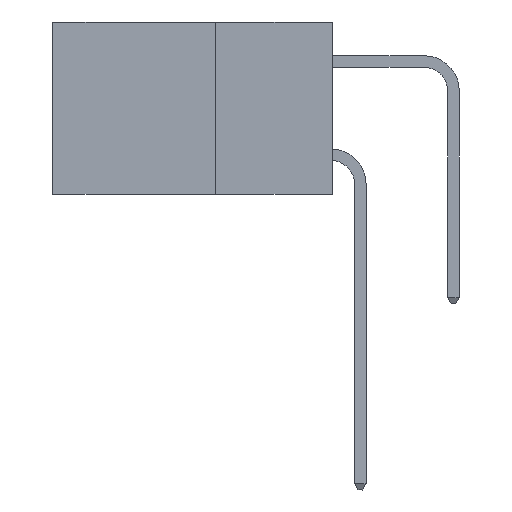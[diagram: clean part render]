
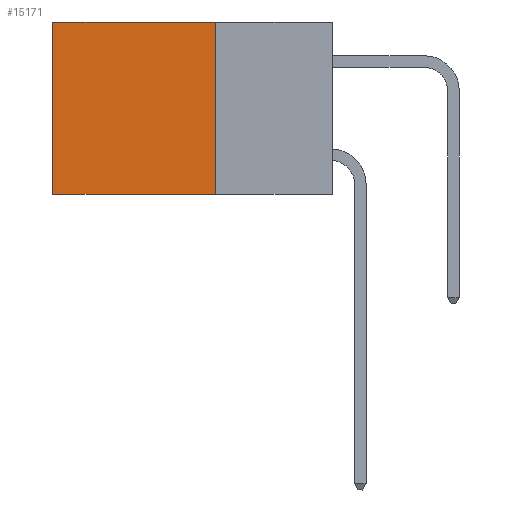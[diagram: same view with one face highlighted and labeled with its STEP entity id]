
A CAD part, left-side view. The second image highlights one B-rep face of the part: STEP entity #15171.
In plain terms, the highlighted planar face has unit normal (-1, 0, 0).
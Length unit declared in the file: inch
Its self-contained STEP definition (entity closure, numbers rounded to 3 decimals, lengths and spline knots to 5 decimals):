
#57 = DIRECTION ( 'NONE',  ( 0., 1., 0. ) ) ;
#191 = CARTESIAN_POINT ( 'NONE',  ( 0.298, 0.25, 0. ) ) ;
#913 = EDGE_CURVE ( 'NONE', #8604, #12734, #20080, .T. ) ;
#1960 = DIRECTION ( 'NONE',  ( 0., 1., 0. ) ) ;
#3022 = ORIENTED_EDGE ( 'NONE', *, *, #7947, .T. ) ;
#3109 = CARTESIAN_POINT ( 'NONE',  ( 0.298, 0.25, 0. ) ) ;
#3699 = VERTEX_POINT ( 'NONE', #13291 ) ;
#3795 = ORIENTED_EDGE ( 'NONE', *, *, #8197, .F. ) ;
#5939 = VERTEX_POINT ( 'NONE', #18798 ) ;
#6107 = LINE ( 'NONE', #9723, #14970 ) ;
#6274 = DIRECTION ( 'NONE',  ( 1., 0., 0. ) ) ;
#7087 = VECTOR ( 'NONE', #57, 39.37008 ) ;
#7766 = PLANE ( 'NONE',  #12631 ) ;
#7947 = EDGE_CURVE ( 'NONE', #5939, #8604, #10801, .T. ) ;
#8197 = EDGE_CURVE ( 'NONE', #5939, #3699, #9546, .T. ) ;
#8595 = EDGE_LOOP ( 'NONE', ( #16766, #17798, #3795, #3022 ) ) ;
#8604 = VERTEX_POINT ( 'NONE', #13914 ) ;
#8838 = EDGE_CURVE ( 'NONE', #3699, #12734, #6107, .T. ) ;
#9516 = CARTESIAN_POINT ( 'NONE',  ( 0.298, 0.6, 0. ) ) ;
#9546 = LINE ( 'NONE', #191, #17985 ) ;
#9723 = CARTESIAN_POINT ( 'NONE',  ( 0.298, 0.25, -0.37 ) ) ;
#9848 = CARTESIAN_POINT ( 'NONE',  ( 0.298, 0.25, 0. ) ) ;
#10801 = LINE ( 'NONE', #9848, #7087 ) ;
#11315 = VECTOR ( 'NONE', #18685, 39.37008 ) ;
#11689 = FACE_OUTER_BOUND ( 'NONE', #8595, .T. ) ;
#12631 = AXIS2_PLACEMENT_3D ( 'NONE', #3109, #6274, #17336 ) ;
#12734 = VERTEX_POINT ( 'NONE', #17383 ) ;
#13291 = CARTESIAN_POINT ( 'NONE',  ( 0.298, 0.25, -0.37 ) ) ;
#13914 = CARTESIAN_POINT ( 'NONE',  ( 0.298, 0.6, 0. ) ) ;
#14970 = VECTOR ( 'NONE', #1960, 39.37008 ) ;
#15171 = ADVANCED_FACE ( 'NONE', ( #11689 ), #7766, .F. ) ;
#15884 = DIRECTION ( 'NONE',  ( 0., 0., -1. ) ) ;
#16766 = ORIENTED_EDGE ( 'NONE', *, *, #913, .T. ) ;
#17336 = DIRECTION ( 'NONE',  ( 0., 0., -1. ) ) ;
#17383 = CARTESIAN_POINT ( 'NONE',  ( 0.298, 0.6, -0.37 ) ) ;
#17798 = ORIENTED_EDGE ( 'NONE', *, *, #8838, .F. ) ;
#17985 = VECTOR ( 'NONE', #15884, 39.37008 ) ;
#18685 = DIRECTION ( 'NONE',  ( 0., 0., -1. ) ) ;
#18798 = CARTESIAN_POINT ( 'NONE',  ( 0.298, 0.25, 0. ) ) ;
#20080 = LINE ( 'NONE', #9516, #11315 ) ;
